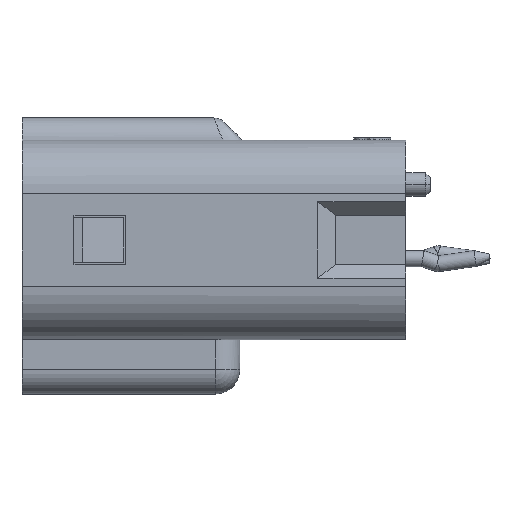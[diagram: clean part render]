
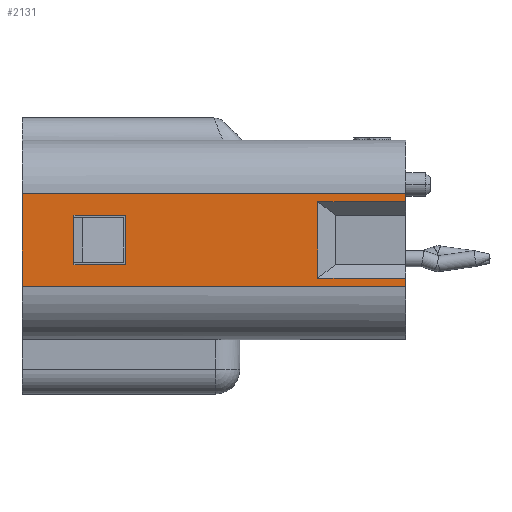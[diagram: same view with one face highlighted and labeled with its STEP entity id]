
A CAD part, left-side view. The second image highlights one B-rep face of the part: STEP entity #2131.
In plain terms, the highlighted planar face has unit normal (-1, 0, 0).
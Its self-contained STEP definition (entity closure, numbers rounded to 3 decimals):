
#750 = DIRECTION ( 'NONE',  ( 0., 0., 1. ) ) ;
#808 = LINE ( 'NONE', #2306, #8440 ) ;
#861 = VECTOR ( 'NONE', #14588, 1000. ) ;
#1188 = VERTEX_POINT ( 'NONE', #8526 ) ;
#1211 = ORIENTED_EDGE ( 'NONE', *, *, #16198, .T. ) ;
#1294 = ORIENTED_EDGE ( 'NONE', *, *, #19497, .T. ) ;
#1558 = DIRECTION ( 'NONE',  ( 0., 0., -1. ) ) ;
#1721 = CARTESIAN_POINT ( 'NONE',  ( -0.1, 10.2, -2.75 ) ) ;
#1939 = CARTESIAN_POINT ( 'NONE',  ( -0.1, 6., -5.625 ) ) ;
#2131 = ADVANCED_FACE ( 'NONE', ( #9090, #17228 ), #6097, .T. ) ;
#2143 = CARTESIAN_POINT ( 'NONE',  ( -0.1, 8.1, -3.625 ) ) ;
#2229 = LINE ( 'NONE', #3732, #14976 ) ;
#2306 = CARTESIAN_POINT ( 'NONE',  ( -0.1, 6., -5.625 ) ) ;
#2414 = CARTESIAN_POINT ( 'NONE',  ( -0.1, 10.2, -2.75 ) ) ;
#2566 = LINE ( 'NONE', #20362, #2981 ) ;
#2644 = CARTESIAN_POINT ( 'NONE',  ( -0.1, -5.3, -6.175 ) ) ;
#2981 = VECTOR ( 'NONE', #750, 1000. ) ;
#3089 = CARTESIAN_POINT ( 'NONE',  ( -0.1, -1.75, -6.175 ) ) ;
#3137 = EDGE_CURVE ( 'NONE', #19386, #17798, #6147, .T. ) ;
#3560 = ORIENTED_EDGE ( 'NONE', *, *, #20258, .F. ) ;
#3732 = CARTESIAN_POINT ( 'NONE',  ( -0.1, 8.1, -3.625 ) ) ;
#4025 = DIRECTION ( 'NONE',  ( 0., 1., 0. ) ) ;
#4273 = VERTEX_POINT ( 'NONE', #1939 ) ;
#4529 = EDGE_LOOP ( 'NONE', ( #15076, #17640, #18031, #1294 ) ) ;
#4794 = EDGE_CURVE ( 'NONE', #13303, #17963, #8857, .T. ) ;
#4888 = CARTESIAN_POINT ( 'NONE',  ( -0.1, -5.3, -6.175 ) ) ;
#4957 = VECTOR ( 'NONE', #8412, 1000. ) ;
#5229 = EDGE_CURVE ( 'NONE', #5468, #4273, #12038, .T. ) ;
#5285 = CARTESIAN_POINT ( 'NONE',  ( -0.1, -5.3, -2.75 ) ) ;
#5390 = EDGE_CURVE ( 'NONE', #18139, #16677, #18110, .T. ) ;
#5434 = VECTOR ( 'NONE', #17268, 1000. ) ;
#5468 = VERTEX_POINT ( 'NONE', #20146 ) ;
#5579 = ORIENTED_EDGE ( 'NONE', *, *, #5390, .F. ) ;
#5606 = VECTOR ( 'NONE', #15385, 1000. ) ;
#5841 = EDGE_CURVE ( 'NONE', #18139, #13303, #14549, .T. ) ;
#5972 = EDGE_LOOP ( 'NONE', ( #15237, #3560, #5579, #7018, #13933, #7988, #15546, #1211 ) ) ;
#6097 = PLANE ( 'NONE',  #15238 ) ;
#6147 = LINE ( 'NONE', #8063, #861 ) ;
#6422 = DIRECTION ( 'NONE',  ( 0., 0., -1. ) ) ;
#7018 = ORIENTED_EDGE ( 'NONE', *, *, #5841, .T. ) ;
#7347 = DIRECTION ( 'NONE',  ( 0., 1., 0. ) ) ;
#7965 = CARTESIAN_POINT ( 'NONE',  ( -0.1, -1.75, -3.075 ) ) ;
#7988 = ORIENTED_EDGE ( 'NONE', *, *, #16754, .F. ) ;
#7989 = LINE ( 'NONE', #4888, #11869 ) ;
#8063 = CARTESIAN_POINT ( 'NONE',  ( -0.1, 8.1, -5.625 ) ) ;
#8211 = CARTESIAN_POINT ( 'NONE',  ( -0.1, -1.75, -3.075 ) ) ;
#8258 = DIRECTION ( 'NONE',  ( 0., -1., 0. ) ) ;
#8412 = DIRECTION ( 'NONE',  ( 0., 0., -1. ) ) ;
#8440 = VECTOR ( 'NONE', #7347, 1000. ) ;
#8526 = CARTESIAN_POINT ( 'NONE',  ( -0.1, -5.3, -3.075 ) ) ;
#8749 = EDGE_CURVE ( 'NONE', #17128, #1188, #9709, .T. ) ;
#8857 = LINE ( 'NONE', #18508, #5606 ) ;
#9090 = FACE_BOUND ( 'NONE', #4529, .T. ) ;
#9709 = LINE ( 'NONE', #8211, #17065 ) ;
#9741 = VECTOR ( 'NONE', #8258, 1000. ) ;
#9849 = VERTEX_POINT ( 'NONE', #3089 ) ;
#10781 = CARTESIAN_POINT ( 'NONE',  ( -0.1, -5.3, -2.75 ) ) ;
#11005 = DIRECTION ( 'NONE',  ( 0., 0., -1. ) ) ;
#11303 = CARTESIAN_POINT ( 'NONE',  ( -0.1, -5.3, -6.5 ) ) ;
#11449 = VECTOR ( 'NONE', #6422, 1000. ) ;
#11869 = VECTOR ( 'NONE', #1558, 1000. ) ;
#12038 = LINE ( 'NONE', #13222, #4957 ) ;
#12147 = CARTESIAN_POINT ( 'NONE',  ( -0.1, -5.3, -6.175 ) ) ;
#12715 = CARTESIAN_POINT ( 'NONE',  ( -0.1, 10.2, -2.75 ) ) ;
#13222 = CARTESIAN_POINT ( 'NONE',  ( -0.1, 6., -3.625 ) ) ;
#13297 = LINE ( 'NONE', #5285, #5434 ) ;
#13303 = VERTEX_POINT ( 'NONE', #20444 ) ;
#13933 = ORIENTED_EDGE ( 'NONE', *, *, #4794, .T. ) ;
#14549 = LINE ( 'NONE', #16156, #11449 ) ;
#14588 = DIRECTION ( 'NONE',  ( 0., 0., 1. ) ) ;
#14976 = VECTOR ( 'NONE', #19809, 1000. ) ;
#15076 = ORIENTED_EDGE ( 'NONE', *, *, #5229, .T. ) ;
#15237 = ORIENTED_EDGE ( 'NONE', *, *, #8749, .T. ) ;
#15238 = AXIS2_PLACEMENT_3D ( 'NONE', #12715, #19159, #11005 ) ;
#15362 = LINE ( 'NONE', #12147, #20090 ) ;
#15385 = DIRECTION ( 'NONE',  ( 0., -1., 0. ) ) ;
#15546 = ORIENTED_EDGE ( 'NONE', *, *, #18221, .T. ) ;
#16156 = CARTESIAN_POINT ( 'NONE',  ( -0.1, 10.2, -2.75 ) ) ;
#16198 = EDGE_CURVE ( 'NONE', #9849, #17128, #2566, .T. ) ;
#16677 = VERTEX_POINT ( 'NONE', #10781 ) ;
#16707 = VERTEX_POINT ( 'NONE', #2644 ) ;
#16754 = EDGE_CURVE ( 'NONE', #16707, #17963, #7989, .T. ) ;
#17065 = VECTOR ( 'NONE', #19362, 1000. ) ;
#17128 = VERTEX_POINT ( 'NONE', #7965 ) ;
#17228 = FACE_OUTER_BOUND ( 'NONE', #5972, .T. ) ;
#17268 = DIRECTION ( 'NONE',  ( 0., 0., -1. ) ) ;
#17640 = ORIENTED_EDGE ( 'NONE', *, *, #18170, .T. ) ;
#17798 = VERTEX_POINT ( 'NONE', #2143 ) ;
#17963 = VERTEX_POINT ( 'NONE', #11303 ) ;
#18031 = ORIENTED_EDGE ( 'NONE', *, *, #3137, .T. ) ;
#18110 = LINE ( 'NONE', #1721, #9741 ) ;
#18139 = VERTEX_POINT ( 'NONE', #2414 ) ;
#18170 = EDGE_CURVE ( 'NONE', #4273, #19386, #808, .T. ) ;
#18221 = EDGE_CURVE ( 'NONE', #16707, #9849, #15362, .T. ) ;
#18508 = CARTESIAN_POINT ( 'NONE',  ( -0.1, 10.2, -6.5 ) ) ;
#19159 = DIRECTION ( 'NONE',  ( -1., 0., 0. ) ) ;
#19362 = DIRECTION ( 'NONE',  ( 0., -1., 0. ) ) ;
#19386 = VERTEX_POINT ( 'NONE', #20996 ) ;
#19497 = EDGE_CURVE ( 'NONE', #17798, #5468, #2229, .T. ) ;
#19809 = DIRECTION ( 'NONE',  ( 0., -1., 0. ) ) ;
#20090 = VECTOR ( 'NONE', #4025, 1000. ) ;
#20146 = CARTESIAN_POINT ( 'NONE',  ( -0.1, 6., -3.625 ) ) ;
#20258 = EDGE_CURVE ( 'NONE', #16677, #1188, #13297, .T. ) ;
#20362 = CARTESIAN_POINT ( 'NONE',  ( -0.1, -1.75, -6.175 ) ) ;
#20444 = CARTESIAN_POINT ( 'NONE',  ( -0.1, 10.2, -6.5 ) ) ;
#20996 = CARTESIAN_POINT ( 'NONE',  ( -0.1, 8.1, -5.625 ) ) ;
